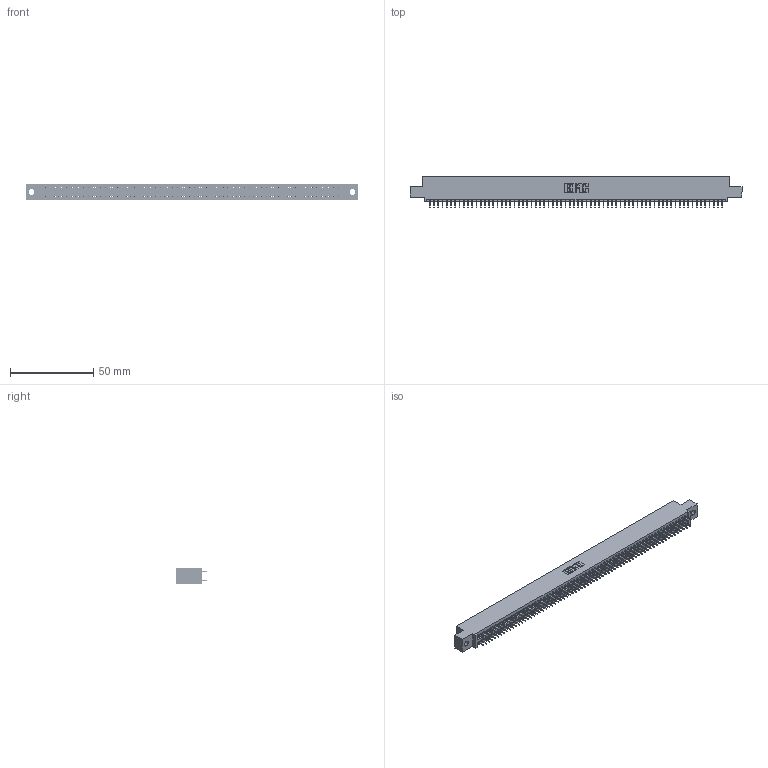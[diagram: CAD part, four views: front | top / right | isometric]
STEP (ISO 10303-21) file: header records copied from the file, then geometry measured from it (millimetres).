
FILE_DESCRIPTION (( 'STEP AP203' ), '1' );
FILE_NAME ('345-140-525-502.STEP', '2020-09-22T17:27:51', ( '' ), ( '' ), 'SwSTEP 2.0', 'SolidWorks 2020', '' );
FILE_SCHEMA (( 'CONFIG_CONTROL_DESIGN' ));
Length unit declared in the file: inch
Products named in the file (3): 345 Part_0.110 Offset - 0.128 Dia; 345-140-525-502; 345-292-001_345-293-125
Assembly tree (141 placements, depth 2):
  345-140-525-502
    345 Part_0.110 Offset - 0.128 Dia
    345-292-001_345-293-125  x140
Bounding box: 199.01 x 18.72 x 9.4 mm (x, y, z)
Volume: 19251.4 mm3; surface area: 28124.7 mm2
Topology: 141 solids, 141 shells, 7690 faces, 21773 edges, 13954 vertices
Faces by surface type: plane 5544, cylinder 2146
Entity records: 51363 total; most frequent: CARTESIAN_POINT 8584, ORIENTED_EDGE 8518, DIRECTION 7535, EDGE_CURVE 4259, LINE 3851, VECTOR 3851, VERTEX_POINT 2834, AXIS2_PLACEMENT_3D 1842
